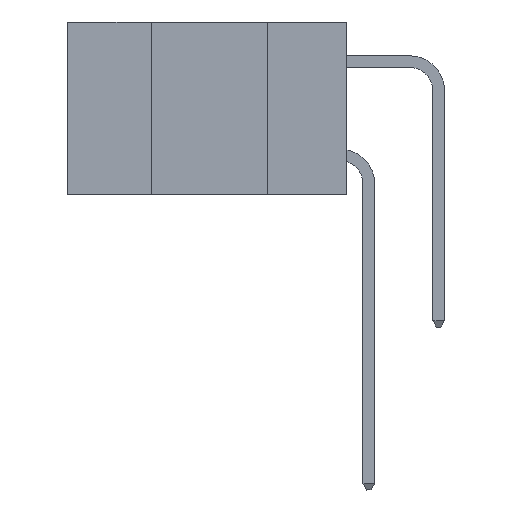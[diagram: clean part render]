
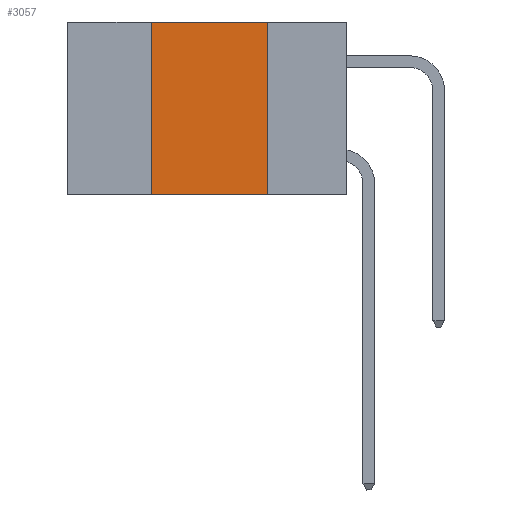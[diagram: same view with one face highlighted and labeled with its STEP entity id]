
A CAD part, left-side view. The second image highlights one B-rep face of the part: STEP entity #3057.
In plain terms, the highlighted planar face has unit normal (-1, 0, 0).
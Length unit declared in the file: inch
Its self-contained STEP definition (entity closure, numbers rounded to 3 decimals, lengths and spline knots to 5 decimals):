
#794 = EDGE_CURVE ( 'NONE', #8336, #15276, #3054, .T. ) ;
#1480 = CARTESIAN_POINT ( 'NONE',  ( 0., 0.42, 0. ) ) ;
#2029 = EDGE_LOOP ( 'NONE', ( #5557, #8195, #19527, #11737 ) ) ;
#3054 = LINE ( 'NONE', #10519, #16394 ) ;
#3057 = ADVANCED_FACE ( 'NONE', ( #4632 ), #10630, .F. ) ;
#3273 = VECTOR ( 'NONE', #19340, 39.37008 ) ;
#3483 = CARTESIAN_POINT ( 'NONE',  ( 0., 0.17, 0. ) ) ;
#3938 = AXIS2_PLACEMENT_3D ( 'NONE', #17707, #12092, #14289 ) ;
#4632 = FACE_OUTER_BOUND ( 'NONE', #2029, .T. ) ;
#4927 = EDGE_CURVE ( 'NONE', #7631, #15276, #22073, .T. ) ;
#5557 = ORIENTED_EDGE ( 'NONE', *, *, #4927, .F. ) ;
#7108 = EDGE_CURVE ( 'NONE', #14654, #7631, #10555, .T. ) ;
#7201 = CARTESIAN_POINT ( 'NONE',  ( 0., 0.17, 0. ) ) ;
#7631 = VERTEX_POINT ( 'NONE', #7201 ) ;
#8195 = ORIENTED_EDGE ( 'NONE', *, *, #7108, .F. ) ;
#8336 = VERTEX_POINT ( 'NONE', #11648 ) ;
#8798 = DIRECTION ( 'NONE',  ( 0., 0., 1. ) ) ;
#9113 = DIRECTION ( 'NONE',  ( 0., 0., -1. ) ) ;
#9549 = VECTOR ( 'NONE', #8798, 39.37008 ) ;
#10519 = CARTESIAN_POINT ( 'NONE',  ( 0., 0.6, -0.37 ) ) ;
#10555 = LINE ( 'NONE', #12012, #3273 ) ;
#10630 = PLANE ( 'NONE',  #3938 ) ;
#11648 = CARTESIAN_POINT ( 'NONE',  ( 0., 0.42, -0.37 ) ) ;
#11737 = ORIENTED_EDGE ( 'NONE', *, *, #794, .T. ) ;
#12012 = CARTESIAN_POINT ( 'NONE',  ( 0., 0.6, 0. ) ) ;
#12092 = DIRECTION ( 'NONE',  ( 1., 0., 0. ) ) ;
#14289 = DIRECTION ( 'NONE',  ( 0., 0., -1. ) ) ;
#14654 = VERTEX_POINT ( 'NONE', #1480 ) ;
#14708 = EDGE_CURVE ( 'NONE', #8336, #14654, #23738, .T. ) ;
#15276 = VERTEX_POINT ( 'NONE', #17048 ) ;
#16394 = VECTOR ( 'NONE', #17962, 39.37008 ) ;
#17048 = CARTESIAN_POINT ( 'NONE',  ( 0., 0.17, -0.37 ) ) ;
#17707 = CARTESIAN_POINT ( 'NONE',  ( 0., 0.6, 0. ) ) ;
#17962 = DIRECTION ( 'NONE',  ( 0., -1., 0. ) ) ;
#18550 = CARTESIAN_POINT ( 'NONE',  ( 0., 0.42, 0. ) ) ;
#19340 = DIRECTION ( 'NONE',  ( 0., -1., 0. ) ) ;
#19527 = ORIENTED_EDGE ( 'NONE', *, *, #14708, .F. ) ;
#21858 = VECTOR ( 'NONE', #9113, 39.37008 ) ;
#22073 = LINE ( 'NONE', #3483, #21858 ) ;
#23738 = LINE ( 'NONE', #18550, #9549 ) ;
